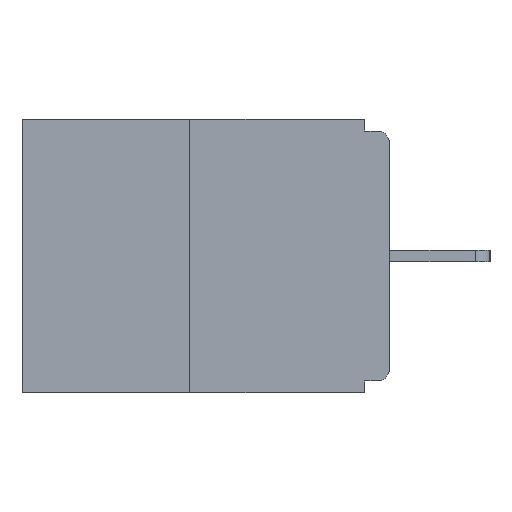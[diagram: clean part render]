
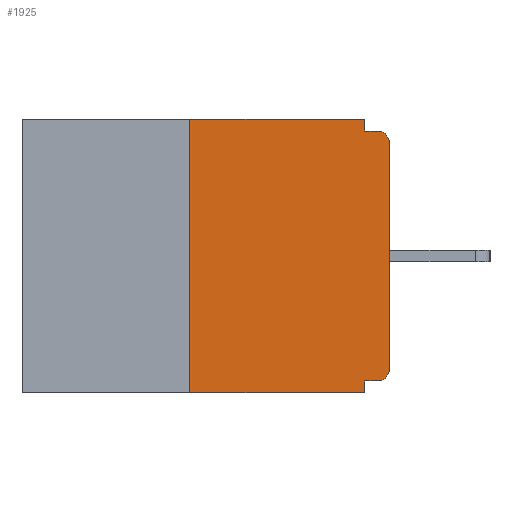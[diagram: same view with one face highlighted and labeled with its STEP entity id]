
A CAD part, left-side view. The second image highlights one B-rep face of the part: STEP entity #1925.
In plain terms, the highlighted planar face has unit normal (-1, 0, 0).
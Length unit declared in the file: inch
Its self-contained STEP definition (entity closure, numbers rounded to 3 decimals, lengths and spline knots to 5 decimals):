
#189 = ORIENTED_EDGE ( 'NONE', *, *, #16814, .F. ) ;
#688 = DIRECTION ( 'NONE',  ( 0., 0., 1. ) ) ;
#917 = LINE ( 'NONE', #3894, #15321 ) ;
#1002 = VECTOR ( 'NONE', #15750, 39.37008 ) ;
#1087 = VECTOR ( 'NONE', #688, 39.37008 ) ;
#1791 = EDGE_CURVE ( 'NONE', #17560, #13634, #8798, .T. ) ;
#1925 = ADVANCED_FACE ( 'NONE', ( #5093 ), #14937, .F. ) ;
#2036 = DIRECTION ( 'NONE',  ( 0., 0., -1. ) ) ;
#2056 = VECTOR ( 'NONE', #16695, 39.37008 ) ;
#2173 = EDGE_LOOP ( 'NONE', ( #6614, #14048, #10784, #3719, #8918, #4465, #2326, #10261, #13518, #189 ) ) ;
#2326 = ORIENTED_EDGE ( 'NONE', *, *, #1791, .T. ) ;
#2520 = VERTEX_POINT ( 'NONE', #3100 ) ;
#2720 = CARTESIAN_POINT ( 'NONE',  ( 0., 0.25, 0. ) ) ;
#2815 = LINE ( 'NONE', #11001, #2056 ) ;
#3100 = CARTESIAN_POINT ( 'NONE',  ( 0., 0.015, -0.328 ) ) ;
#3302 = LINE ( 'NONE', #6165, #1002 ) ;
#3517 = CARTESIAN_POINT ( 'NONE',  ( 0., 0.031, -0.015 ) ) ;
#3563 = VECTOR ( 'NONE', #11059, 39.37008 ) ;
#3610 = CARTESIAN_POINT ( 'NONE',  ( 0., 0.031, 0. ) ) ;
#3719 = ORIENTED_EDGE ( 'NONE', *, *, #14860, .F. ) ;
#3884 = VERTEX_POINT ( 'NONE', #12075 ) ;
#3888 = VERTEX_POINT ( 'NONE', #3517 ) ;
#3894 = CARTESIAN_POINT ( 'NONE',  ( 0., 0.031, -0.343 ) ) ;
#4465 = ORIENTED_EDGE ( 'NONE', *, *, #4721, .T. ) ;
#4570 = EDGE_CURVE ( 'NONE', #13634, #8244, #13212, .T. ) ;
#4721 = EDGE_CURVE ( 'NONE', #2520, #17560, #13231, .T. ) ;
#4870 = VERTEX_POINT ( 'NONE', #13471 ) ;
#4995 = CARTESIAN_POINT ( 'NONE',  ( 0., 0.015, -0.313 ) ) ;
#5093 = FACE_OUTER_BOUND ( 'NONE', #2173, .T. ) ;
#5113 = CARTESIAN_POINT ( 'NONE',  ( 0., 0., -0.015 ) ) ;
#5461 = AXIS2_PLACEMENT_3D ( 'NONE', #4995, #15920, #2036 ) ;
#6165 = CARTESIAN_POINT ( 'NONE',  ( 0., 0.031, 0. ) ) ;
#6489 = EDGE_CURVE ( 'NONE', #3884, #4870, #6768, .T. ) ;
#6614 = ORIENTED_EDGE ( 'NONE', *, *, #15848, .F. ) ;
#6768 = LINE ( 'NONE', #16354, #12268 ) ;
#6795 = DIRECTION ( 'NONE',  ( 0., 0., -1. ) ) ;
#6806 = VERTEX_POINT ( 'NONE', #3610 ) ;
#8244 = VERTEX_POINT ( 'NONE', #11426 ) ;
#8747 = CARTESIAN_POINT ( 'NONE',  ( 0., 0., -0.328 ) ) ;
#8798 = LINE ( 'NONE', #9060, #1087 ) ;
#8918 = ORIENTED_EDGE ( 'NONE', *, *, #17553, .F. ) ;
#9060 = CARTESIAN_POINT ( 'NONE',  ( 0., 0., 0. ) ) ;
#9326 = CARTESIAN_POINT ( 'NONE',  ( 0., 0.46, 0. ) ) ;
#9471 = DIRECTION ( 'NONE',  ( 0., -1., 0. ) ) ;
#9701 = AXIS2_PLACEMENT_3D ( 'NONE', #9326, #17649, #6795 ) ;
#9872 = DIRECTION ( 'NONE',  ( 0., 0., -1. ) ) ;
#10013 = LINE ( 'NONE', #15432, #15662 ) ;
#10261 = ORIENTED_EDGE ( 'NONE', *, *, #4570, .T. ) ;
#10331 = VERTEX_POINT ( 'NONE', #12639 ) ;
#10738 = CARTESIAN_POINT ( 'NONE',  ( 0., 0., -0.03 ) ) ;
#10779 = VECTOR ( 'NONE', #15532, 39.37008 ) ;
#10784 = ORIENTED_EDGE ( 'NONE', *, *, #6489, .T. ) ;
#11001 = CARTESIAN_POINT ( 'NONE',  ( 0., 0.25, 0. ) ) ;
#11059 = DIRECTION ( 'NONE',  ( 0., -1., 0. ) ) ;
#11426 = CARTESIAN_POINT ( 'NONE',  ( 0., 0.015, -0.015 ) ) ;
#11623 = CARTESIAN_POINT ( 'NONE',  ( 0., 0., -0.313 ) ) ;
#11962 = LINE ( 'NONE', #5113, #3563 ) ;
#12075 = CARTESIAN_POINT ( 'NONE',  ( 0., 0.25, -0.343 ) ) ;
#12096 = DIRECTION ( 'NONE',  ( 0., 0., -1. ) ) ;
#12268 = VECTOR ( 'NONE', #9471, 39.37008 ) ;
#12639 = CARTESIAN_POINT ( 'NONE',  ( 0., 0.031, -0.328 ) ) ;
#12826 = DIRECTION ( 'NONE',  ( -1., 0., 0. ) ) ;
#13212 = CIRCLE ( 'NONE', #15538, 0.015 ) ;
#13231 = CIRCLE ( 'NONE', #5461, 0.015 ) ;
#13471 = CARTESIAN_POINT ( 'NONE',  ( 0., 0.031, -0.343 ) ) ;
#13518 = ORIENTED_EDGE ( 'NONE', *, *, #16625, .F. ) ;
#13634 = VERTEX_POINT ( 'NONE', #10738 ) ;
#13714 = EDGE_CURVE ( 'NONE', #3884, #13802, #2815, .T. ) ;
#13802 = VERTEX_POINT ( 'NONE', #2720 ) ;
#14048 = ORIENTED_EDGE ( 'NONE', *, *, #13714, .F. ) ;
#14208 = CARTESIAN_POINT ( 'NONE',  ( 0., 0.015, -0.03 ) ) ;
#14860 = EDGE_CURVE ( 'NONE', #10331, #4870, #917, .T. ) ;
#14937 = PLANE ( 'NONE',  #9701 ) ;
#15321 = VECTOR ( 'NONE', #12096, 39.37008 ) ;
#15432 = CARTESIAN_POINT ( 'NONE',  ( 0., 0.46, 0. ) ) ;
#15532 = DIRECTION ( 'NONE',  ( 0., 1., 0. ) ) ;
#15538 = AXIS2_PLACEMENT_3D ( 'NONE', #14208, #12826, #9872 ) ;
#15662 = VECTOR ( 'NONE', #16620, 39.37008 ) ;
#15750 = DIRECTION ( 'NONE',  ( 0., 0., -1. ) ) ;
#15848 = EDGE_CURVE ( 'NONE', #13802, #6806, #10013, .T. ) ;
#15920 = DIRECTION ( 'NONE',  ( -1., 0., 0. ) ) ;
#16354 = CARTESIAN_POINT ( 'NONE',  ( 0., 0.46, -0.343 ) ) ;
#16620 = DIRECTION ( 'NONE',  ( 0., -1., 0. ) ) ;
#16625 = EDGE_CURVE ( 'NONE', #3888, #8244, #11962, .T. ) ;
#16695 = DIRECTION ( 'NONE',  ( 0., 0., 1. ) ) ;
#16814 = EDGE_CURVE ( 'NONE', #6806, #3888, #3302, .T. ) ;
#16887 = LINE ( 'NONE', #8747, #10779 ) ;
#17553 = EDGE_CURVE ( 'NONE', #2520, #10331, #16887, .T. ) ;
#17560 = VERTEX_POINT ( 'NONE', #11623 ) ;
#17649 = DIRECTION ( 'NONE',  ( 1., 0., 0. ) ) ;
